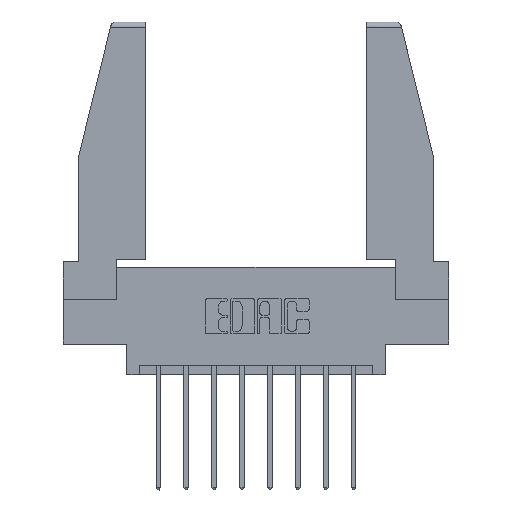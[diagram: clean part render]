
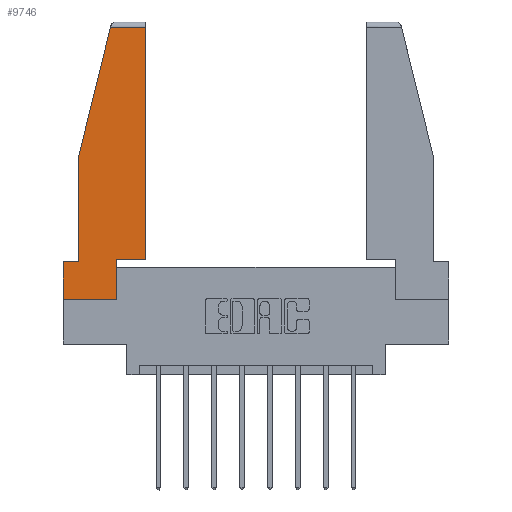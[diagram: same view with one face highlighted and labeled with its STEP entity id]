
A CAD part, top view. The second image highlights one B-rep face of the part: STEP entity #9746.
In plain terms, the highlighted planar face has unit normal (0, 0, 1).
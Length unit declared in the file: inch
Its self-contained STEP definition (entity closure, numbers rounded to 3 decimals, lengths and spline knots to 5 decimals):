
#270 = ORIENTED_EDGE ( 'NONE', *, *, #11665, .T. ) ;
#326 = ORIENTED_EDGE ( 'NONE', *, *, #7786, .T. ) ;
#372 = PLANE ( 'NONE',  #11473 ) ;
#440 = VECTOR ( 'NONE', #1593, 39.37008 ) ;
#859 = EDGE_CURVE ( 'NONE', #2876, #8628, #3655, .T. ) ;
#875 = CARTESIAN_POINT ( 'NONE',  ( 0.461, 1.52, 0. ) ) ;
#1130 = VERTEX_POINT ( 'NONE', #10205 ) ;
#1186 = VERTEX_POINT ( 'NONE', #7277 ) ;
#1319 = VECTOR ( 'NONE', #8557, 39.37008 ) ;
#1337 = CARTESIAN_POINT ( 'NONE',  ( 0.461, 0.223, 0. ) ) ;
#1404 = DIRECTION ( 'NONE',  ( 1., 0., 0. ) ) ;
#1593 = DIRECTION ( 'NONE',  ( 0., -1., 0. ) ) ;
#1712 = CARTESIAN_POINT ( 'NONE',  ( 0., 1.52, 0. ) ) ;
#1922 = VECTOR ( 'NONE', #4719, 39.37008 ) ;
#2317 = FACE_OUTER_BOUND ( 'NONE', #6064, .T. ) ;
#2394 = CARTESIAN_POINT ( 'NONE',  ( 0.297, 0., 0. ) ) ;
#2582 = CARTESIAN_POINT ( 'NONE',  ( 0., 0.21, 0. ) ) ;
#2621 = CARTESIAN_POINT ( 'NONE',  ( 0., 0., 0. ) ) ;
#2798 = VECTOR ( 'NONE', #6213, 39.37008 ) ;
#2876 = VERTEX_POINT ( 'NONE', #875 ) ;
#3123 = VECTOR ( 'NONE', #11216, 39.37008 ) ;
#3195 = VERTEX_POINT ( 'NONE', #11509 ) ;
#3274 = CARTESIAN_POINT ( 'NONE',  ( 0.271, 1.55, 0. ) ) ;
#3492 = CARTESIAN_POINT ( 'NONE',  ( 0.086, 0.8, 0. ) ) ;
#3556 = VERTEX_POINT ( 'NONE', #11671 ) ;
#3575 = LINE ( 'NONE', #3274, #5973 ) ;
#3655 = LINE ( 'NONE', #1712, #1922 ) ;
#4159 = CARTESIAN_POINT ( 'NONE',  ( 0., 0.21, 0. ) ) ;
#4719 = DIRECTION ( 'NONE',  ( -1., 0., 0. ) ) ;
#5068 = CARTESIAN_POINT ( 'NONE',  ( 0.297, 0.223, 0. ) ) ;
#5156 = EDGE_CURVE ( 'NONE', #12143, #1130, #5820, .T. ) ;
#5721 = DIRECTION ( 'NONE',  ( 0., -1., 0. ) ) ;
#5781 = EDGE_CURVE ( 'NONE', #8628, #3556, #3575, .T. ) ;
#5820 = LINE ( 'NONE', #9985, #3123 ) ;
#5973 = VECTOR ( 'NONE', #6358, 39.37008 ) ;
#5996 = CARTESIAN_POINT ( 'NONE',  ( 0.2636, 1.52, 0. ) ) ;
#6064 = EDGE_LOOP ( 'NONE', ( #10070, #6453, #11210, #12600, #9434, #326, #8047, #270, #6333 ) ) ;
#6213 = DIRECTION ( 'NONE',  ( 0., 1., 0. ) ) ;
#6333 = ORIENTED_EDGE ( 'NONE', *, *, #5156, .T. ) ;
#6358 = DIRECTION ( 'NONE',  ( -0.239, -0.971, 0. ) ) ;
#6443 = VERTEX_POINT ( 'NONE', #4159 ) ;
#6453 = ORIENTED_EDGE ( 'NONE', *, *, #859, .T. ) ;
#7277 = CARTESIAN_POINT ( 'NONE',  ( 0.297, 0., 0. ) ) ;
#7368 = LINE ( 'NONE', #2394, #1319 ) ;
#7786 = EDGE_CURVE ( 'NONE', #6443, #3195, #9517, .T. ) ;
#8047 = ORIENTED_EDGE ( 'NONE', *, *, #11060, .T. ) ;
#8048 = VECTOR ( 'NONE', #9397, 39.37008 ) ;
#8059 = LINE ( 'NONE', #1337, #2798 ) ;
#8361 = EDGE_CURVE ( 'NONE', #3556, #8858, #12708, .T. ) ;
#8557 = DIRECTION ( 'NONE',  ( 0., 1., 0. ) ) ;
#8628 = VERTEX_POINT ( 'NONE', #5996 ) ;
#8826 = EDGE_CURVE ( 'NONE', #1130, #2876, #8059, .T. ) ;
#8858 = VERTEX_POINT ( 'NONE', #9509 ) ;
#9290 = LINE ( 'NONE', #2621, #13146 ) ;
#9397 = DIRECTION ( 'NONE',  ( -1., 0., 0. ) ) ;
#9434 = ORIENTED_EDGE ( 'NONE', *, *, #9686, .T. ) ;
#9509 = CARTESIAN_POINT ( 'NONE',  ( 0.086, 0.21, 0. ) ) ;
#9517 = LINE ( 'NONE', #2582, #440 ) ;
#9530 = DIRECTION ( 'NONE',  ( 0., 0., 1. ) ) ;
#9686 = EDGE_CURVE ( 'NONE', #8858, #6443, #10765, .T. ) ;
#9746 = ADVANCED_FACE ( 'NONE', ( #2317 ), #372, .T. ) ;
#9985 = CARTESIAN_POINT ( 'NONE',  ( 0.297, 0.223, 0. ) ) ;
#10070 = ORIENTED_EDGE ( 'NONE', *, *, #8826, .T. ) ;
#10205 = CARTESIAN_POINT ( 'NONE',  ( 0.461, 0.223, 0. ) ) ;
#10723 = DIRECTION ( 'NONE',  ( 1., 0., 0. ) ) ;
#10765 = LINE ( 'NONE', #12386, #8048 ) ;
#11060 = EDGE_CURVE ( 'NONE', #3195, #1186, #9290, .T. ) ;
#11127 = VECTOR ( 'NONE', #5721, 39.37008 ) ;
#11210 = ORIENTED_EDGE ( 'NONE', *, *, #5781, .T. ) ;
#11216 = DIRECTION ( 'NONE',  ( 1., 0., 0. ) ) ;
#11473 = AXIS2_PLACEMENT_3D ( 'NONE', #12714, #9530, #1404 ) ;
#11509 = CARTESIAN_POINT ( 'NONE',  ( 0., 0., 0. ) ) ;
#11665 = EDGE_CURVE ( 'NONE', #1186, #12143, #7368, .T. ) ;
#11671 = CARTESIAN_POINT ( 'NONE',  ( 0.086, 0.8, 0. ) ) ;
#12143 = VERTEX_POINT ( 'NONE', #5068 ) ;
#12386 = CARTESIAN_POINT ( 'NONE',  ( 0., 0.21, 0. ) ) ;
#12600 = ORIENTED_EDGE ( 'NONE', *, *, #8361, .T. ) ;
#12708 = LINE ( 'NONE', #3492, #11127 ) ;
#12714 = CARTESIAN_POINT ( 'NONE',  ( 0., 0., 0. ) ) ;
#13146 = VECTOR ( 'NONE', #10723, 39.37008 ) ;
